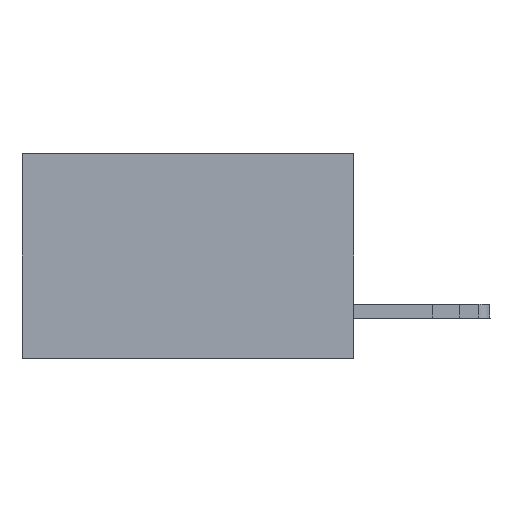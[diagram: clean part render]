
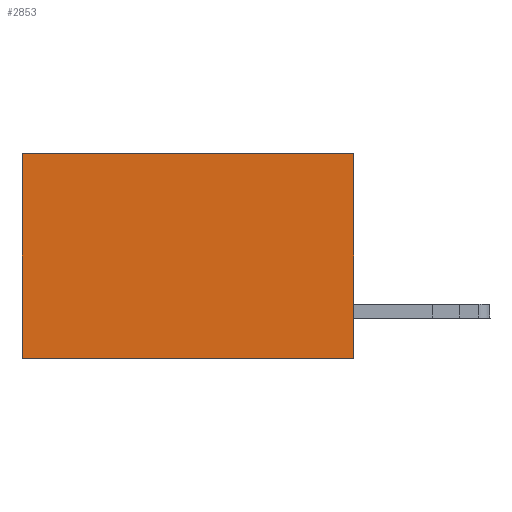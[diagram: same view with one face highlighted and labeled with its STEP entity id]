
A CAD part, left-side view. The second image highlights one B-rep face of the part: STEP entity #2853.
In plain terms, the highlighted planar face has unit normal (-1, 0, 0).
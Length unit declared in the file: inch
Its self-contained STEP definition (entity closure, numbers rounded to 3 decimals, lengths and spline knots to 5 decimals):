
#527 = VERTEX_POINT ( 'NONE', #6499 ) ;
#763 = CARTESIAN_POINT ( 'NONE',  ( 0.2875, 0.6, 0. ) ) ;
#2565 = VECTOR ( 'NONE', #3591, 39.37008 ) ;
#2853 = ADVANCED_FACE ( 'NONE', ( #32151 ), #7171, .F. ) ;
#3591 = DIRECTION ( 'NONE',  ( 0., 1., 0. ) ) ;
#3795 = VERTEX_POINT ( 'NONE', #30868 ) ;
#4043 = ORIENTED_EDGE ( 'NONE', *, *, #22841, .T. ) ;
#4679 = LINE ( 'NONE', #23341, #18566 ) ;
#6499 = CARTESIAN_POINT ( 'NONE',  ( 0.2875, 0., -0.37 ) ) ;
#6557 = LINE ( 'NONE', #763, #19572 ) ;
#6819 = DIRECTION ( 'NONE',  ( 1., 0., 0. ) ) ;
#7171 = PLANE ( 'NONE',  #24130 ) ;
#7917 = DIRECTION ( 'NONE',  ( 0., 0., -1. ) ) ;
#8128 = CARTESIAN_POINT ( 'NONE',  ( 0.2875, 0., 0. ) ) ;
#8403 = EDGE_CURVE ( 'NONE', #15965, #527, #4679, .T. ) ;
#8678 = EDGE_CURVE ( 'NONE', #527, #27551, #16514, .T. ) ;
#13014 = CARTESIAN_POINT ( 'NONE',  ( 0.2875, 0., 0. ) ) ;
#15965 = VERTEX_POINT ( 'NONE', #22062 ) ;
#16514 = LINE ( 'NONE', #21772, #2565 ) ;
#18566 = VECTOR ( 'NONE', #7917, 39.37008 ) ;
#19572 = VECTOR ( 'NONE', #26733, 39.37008 ) ;
#21014 = DIRECTION ( 'NONE',  ( 0., 0., -1. ) ) ;
#21772 = CARTESIAN_POINT ( 'NONE',  ( 0.2875, 0., -0.37 ) ) ;
#22062 = CARTESIAN_POINT ( 'NONE',  ( 0.2875, 0., 0. ) ) ;
#22841 = EDGE_CURVE ( 'NONE', #3795, #27551, #6557, .T. ) ;
#23341 = CARTESIAN_POINT ( 'NONE',  ( 0.2875, 0., 0. ) ) ;
#24130 = AXIS2_PLACEMENT_3D ( 'NONE', #13014, #6819, #21014 ) ;
#24956 = EDGE_LOOP ( 'NONE', ( #4043, #30326, #25997, #26458 ) ) ;
#25997 = ORIENTED_EDGE ( 'NONE', *, *, #8403, .F. ) ;
#26166 = VECTOR ( 'NONE', #30957, 39.37008 ) ;
#26458 = ORIENTED_EDGE ( 'NONE', *, *, #31138, .T. ) ;
#26733 = DIRECTION ( 'NONE',  ( 0., 0., -1. ) ) ;
#27551 = VERTEX_POINT ( 'NONE', #28704 ) ;
#28704 = CARTESIAN_POINT ( 'NONE',  ( 0.2875, 0.6, -0.37 ) ) ;
#30326 = ORIENTED_EDGE ( 'NONE', *, *, #8678, .F. ) ;
#30868 = CARTESIAN_POINT ( 'NONE',  ( 0.2875, 0.6, 0. ) ) ;
#30957 = DIRECTION ( 'NONE',  ( 0., 1., 0. ) ) ;
#31138 = EDGE_CURVE ( 'NONE', #15965, #3795, #32710, .T. ) ;
#32151 = FACE_OUTER_BOUND ( 'NONE', #24956, .T. ) ;
#32710 = LINE ( 'NONE', #8128, #26166 ) ;
